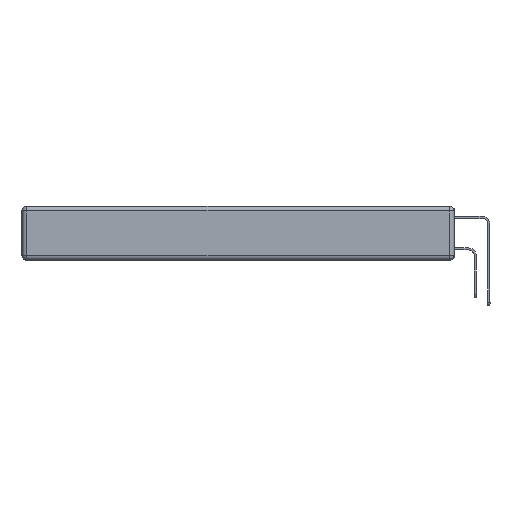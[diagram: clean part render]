
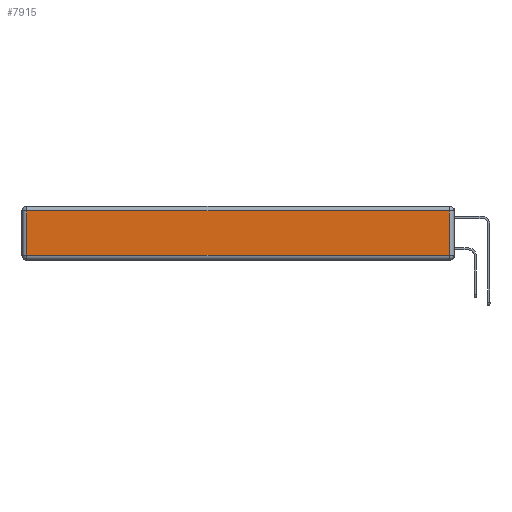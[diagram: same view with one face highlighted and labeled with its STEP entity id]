
A CAD part, left-side view. The second image highlights one B-rep face of the part: STEP entity #7915.
In plain terms, the highlighted planar face has unit normal (-1, 0, 0).
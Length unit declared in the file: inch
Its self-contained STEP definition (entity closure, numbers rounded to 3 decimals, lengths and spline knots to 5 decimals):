
#219 = FACE_OUTER_BOUND ( 'NONE', #11628, .T. ) ;
#1722 = EDGE_CURVE ( 'NONE', #8746, #2404, #7064, .T. ) ;
#2404 = VERTEX_POINT ( 'NONE', #8773 ) ;
#2540 = AXIS2_PLACEMENT_3D ( 'NONE', #11734, #19341, #17533 ) ;
#3145 = ORIENTED_EDGE ( 'NONE', *, *, #11740, .T. ) ;
#5417 = CARTESIAN_POINT ( 'NONE',  ( 0., 2.72, -0.313 ) ) ;
#5643 = VERTEX_POINT ( 'NONE', #14915 ) ;
#5970 = CARTESIAN_POINT ( 'NONE',  ( 0., 2.75, -0.03 ) ) ;
#6434 = ORIENTED_EDGE ( 'NONE', *, *, #1722, .T. ) ;
#7064 = LINE ( 'NONE', #11046, #13523 ) ;
#7845 = VECTOR ( 'NONE', #13596, 39.37008 ) ;
#7915 = ADVANCED_FACE ( 'NONE', ( #219 ), #8108, .T. ) ;
#8108 = PLANE ( 'NONE',  #2540 ) ;
#8746 = VERTEX_POINT ( 'NONE', #23744 ) ;
#8773 = CARTESIAN_POINT ( 'NONE',  ( 0., 0.03, -0.03 ) ) ;
#11046 = CARTESIAN_POINT ( 'NONE',  ( 0., 0.03, -0.343 ) ) ;
#11496 = ORIENTED_EDGE ( 'NONE', *, *, #19824, .T. ) ;
#11628 = EDGE_LOOP ( 'NONE', ( #11496, #6434, #3145, #13694 ) ) ;
#11734 = CARTESIAN_POINT ( 'NONE',  ( 0., 0., -0.343 ) ) ;
#11740 = EDGE_CURVE ( 'NONE', #2404, #5643, #23517, .T. ) ;
#11834 = VERTEX_POINT ( 'NONE', #5417 ) ;
#13441 = LINE ( 'NONE', #24792, #22755 ) ;
#13523 = VECTOR ( 'NONE', #17247, 39.37008 ) ;
#13596 = DIRECTION ( 'NONE',  ( 0., 1., 0. ) ) ;
#13694 = ORIENTED_EDGE ( 'NONE', *, *, #15919, .T. ) ;
#14915 = CARTESIAN_POINT ( 'NONE',  ( 0., 2.72, -0.03 ) ) ;
#14997 = DIRECTION ( 'NONE',  ( 0., 0., -1. ) ) ;
#15919 = EDGE_CURVE ( 'NONE', #5643, #11834, #13441, .T. ) ;
#16287 = DIRECTION ( 'NONE',  ( 0., -1., 0. ) ) ;
#17184 = VECTOR ( 'NONE', #16287, 39.37008 ) ;
#17247 = DIRECTION ( 'NONE',  ( 0., 0., 1. ) ) ;
#17533 = DIRECTION ( 'NONE',  ( 0., 0., 1. ) ) ;
#18090 = CARTESIAN_POINT ( 'NONE',  ( 0., 0., -0.313 ) ) ;
#19341 = DIRECTION ( 'NONE',  ( -1., 0., 0. ) ) ;
#19824 = EDGE_CURVE ( 'NONE', #11834, #8746, #24268, .T. ) ;
#22755 = VECTOR ( 'NONE', #14997, 39.37008 ) ;
#23517 = LINE ( 'NONE', #5970, #7845 ) ;
#23744 = CARTESIAN_POINT ( 'NONE',  ( 0., 0.03, -0.313 ) ) ;
#24268 = LINE ( 'NONE', #18090, #17184 ) ;
#24792 = CARTESIAN_POINT ( 'NONE',  ( 0., 2.72, -0.343 ) ) ;
